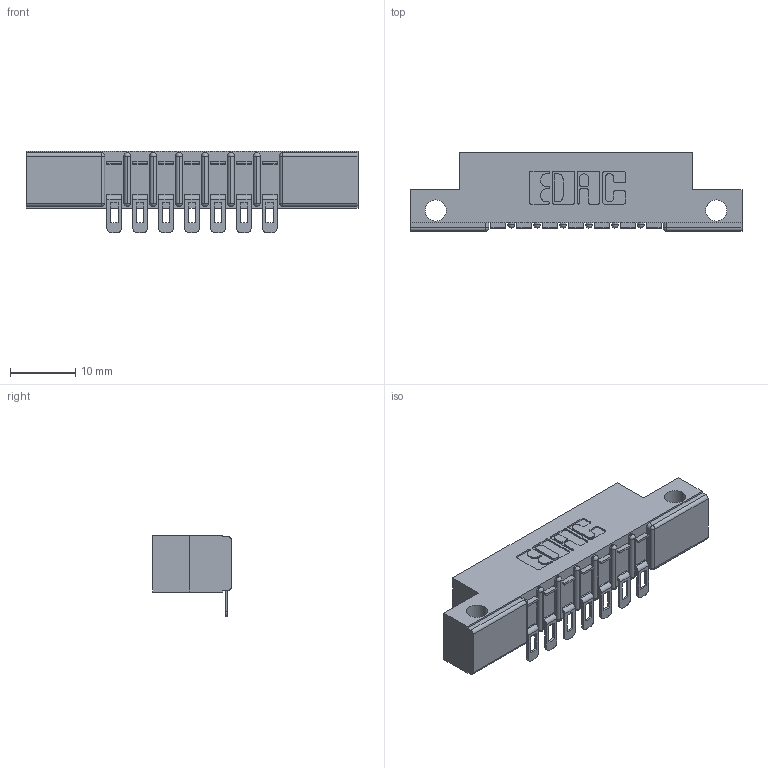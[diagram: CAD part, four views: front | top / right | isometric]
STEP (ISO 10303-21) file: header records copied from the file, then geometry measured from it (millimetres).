
FILE_DESCRIPTION (( 'STEP AP203' ), '1' );
FILE_NAME ('357-007-554-112.STEP', '2018-08-07T00:17:41', ( '' ), ( '' ), 'SwSTEP 2.0', 'SolidWorks 2016', '' );
FILE_SCHEMA (( 'CONFIG_CONTROL_DESIGN' ));
Length unit declared in the file: inch
Products named in the file (3): 307 Part_.128 Dia Side Mounting Holes; 307-290-002_554; 357-007-554-112
Assembly tree (8 placements, depth 2):
  357-007-554-112
    307 Part_.128 Dia Side Mounting Holes
    307-290-002_554  x7
Bounding box: 50.75 x 12.01 x 12.52 mm (x, y, z)
Volume: 3269.1 mm3; surface area: 5003.2 mm2
Topology: 8 solids, 8 shells, 693 faces, 2094 edges, 1372 vertices
Faces by surface type: plane 392, cylinder 285, sphere 16
Entity records: 11283 total; most frequent: CARTESIAN_POINT 1898, ORIENTED_EDGE 1888, DIRECTION 1866, EDGE_CURVE 944, VECTOR 698, LINE 698, VERTEX_POINT 616, AXIS2_PLACEMENT_3D 584
